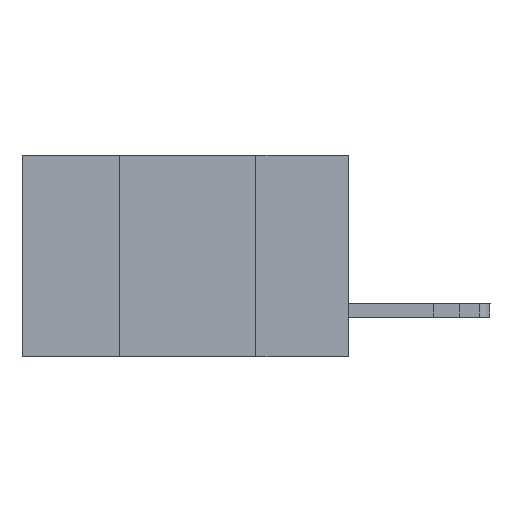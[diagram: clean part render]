
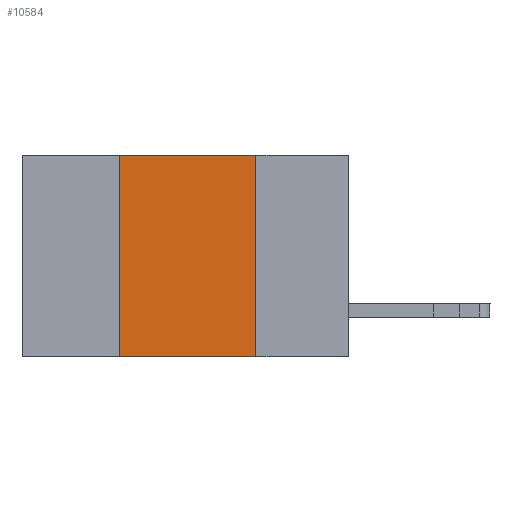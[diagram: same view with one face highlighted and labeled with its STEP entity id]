
A CAD part, left-side view. The second image highlights one B-rep face of the part: STEP entity #10584.
In plain terms, the highlighted planar face has unit normal (-1, 0, 0).
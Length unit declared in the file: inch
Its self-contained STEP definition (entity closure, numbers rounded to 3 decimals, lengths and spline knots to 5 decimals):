
#325 = VECTOR ( 'NONE', #589, 39.37008 ) ;
#571 = CARTESIAN_POINT ( 'NONE',  ( 0., 0.42, -0.37 ) ) ;
#589 = DIRECTION ( 'NONE',  ( 0., -1., 0. ) ) ;
#1036 = EDGE_CURVE ( 'NONE', #11515, #8128, #4061, .T. ) ;
#1639 = LINE ( 'NONE', #12489, #7032 ) ;
#1653 = LINE ( 'NONE', #8571, #7044 ) ;
#1707 = FACE_OUTER_BOUND ( 'NONE', #9046, .T. ) ;
#2074 = EDGE_CURVE ( 'NONE', #11515, #12238, #1653, .T. ) ;
#2534 = EDGE_CURVE ( 'NONE', #11207, #12238, #1639, .T. ) ;
#2927 = PLANE ( 'NONE',  #11090 ) ;
#3222 = DIRECTION ( 'NONE',  ( 0., -1., 0. ) ) ;
#4061 = LINE ( 'NONE', #571, #6552 ) ;
#4398 = ORIENTED_EDGE ( 'NONE', *, *, #1036, .F. ) ;
#6552 = VECTOR ( 'NONE', #10036, 39.37008 ) ;
#7032 = VECTOR ( 'NONE', #12625, 39.37008 ) ;
#7044 = VECTOR ( 'NONE', #3222, 39.37008 ) ;
#7238 = DIRECTION ( 'NONE',  ( 0., 0., -1. ) ) ;
#7408 = CARTESIAN_POINT ( 'NONE',  ( 0., 0.17, 0. ) ) ;
#7443 = ORIENTED_EDGE ( 'NONE', *, *, #2074, .T. ) ;
#8128 = VERTEX_POINT ( 'NONE', #12343 ) ;
#8239 = ORIENTED_EDGE ( 'NONE', *, *, #9816, .F. ) ;
#8571 = CARTESIAN_POINT ( 'NONE',  ( 0., 0.6, -0.37 ) ) ;
#8635 = LINE ( 'NONE', #13494, #325 ) ;
#9046 = EDGE_LOOP ( 'NONE', ( #12649, #8239, #4398, #7443 ) ) ;
#9816 = EDGE_CURVE ( 'NONE', #8128, #11207, #8635, .T. ) ;
#10036 = DIRECTION ( 'NONE',  ( 0., 0., 1. ) ) ;
#10100 = CARTESIAN_POINT ( 'NONE',  ( 0., 0.42, -0.37 ) ) ;
#10348 = CARTESIAN_POINT ( 'NONE',  ( 0., 0.17, -0.37 ) ) ;
#10584 = ADVANCED_FACE ( 'NONE', ( #1707 ), #2927, .F. ) ;
#11090 = AXIS2_PLACEMENT_3D ( 'NONE', #12594, #13651, #7238 ) ;
#11207 = VERTEX_POINT ( 'NONE', #7408 ) ;
#11515 = VERTEX_POINT ( 'NONE', #10100 ) ;
#12238 = VERTEX_POINT ( 'NONE', #10348 ) ;
#12343 = CARTESIAN_POINT ( 'NONE',  ( 0., 0.42, 0. ) ) ;
#12489 = CARTESIAN_POINT ( 'NONE',  ( 0., 0.17, -0.37 ) ) ;
#12594 = CARTESIAN_POINT ( 'NONE',  ( 0., 0.6, 0. ) ) ;
#12625 = DIRECTION ( 'NONE',  ( 0., 0., -1. ) ) ;
#12649 = ORIENTED_EDGE ( 'NONE', *, *, #2534, .F. ) ;
#13494 = CARTESIAN_POINT ( 'NONE',  ( 0., 0.6, 0. ) ) ;
#13651 = DIRECTION ( 'NONE',  ( 1., 0., 0. ) ) ;
